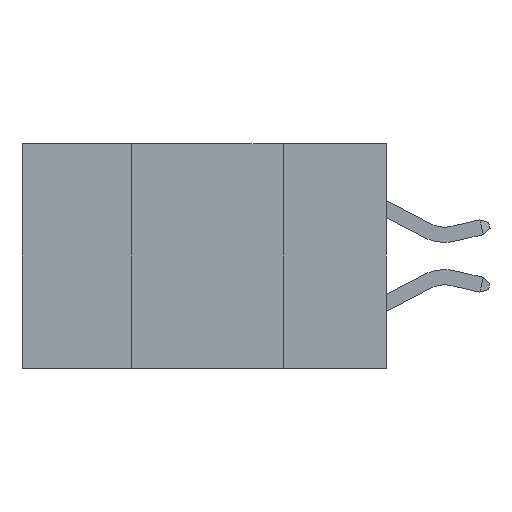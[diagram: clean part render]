
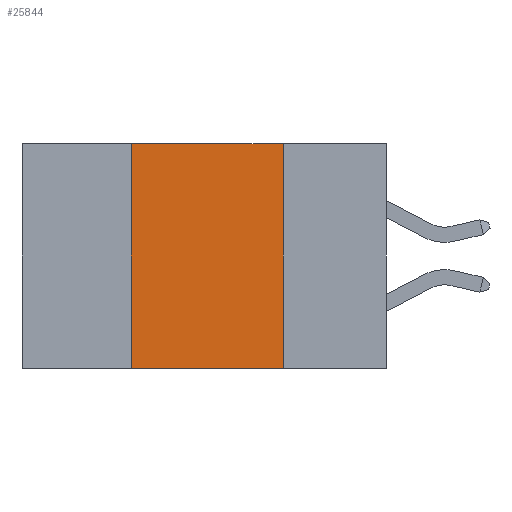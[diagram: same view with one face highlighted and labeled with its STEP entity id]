
A CAD part, left-side view. The second image highlights one B-rep face of the part: STEP entity #25844.
In plain terms, the highlighted planar face has unit normal (-1, 0, 0).
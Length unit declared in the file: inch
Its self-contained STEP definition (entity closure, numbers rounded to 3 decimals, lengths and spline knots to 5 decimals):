
#2453 = CARTESIAN_POINT ( 'NONE',  ( 0., 0.42, 0. ) ) ;
#2692 = VERTEX_POINT ( 'NONE', #3532 ) ;
#3270 = ORIENTED_EDGE ( 'NONE', *, *, #11109, .F. ) ;
#3532 = CARTESIAN_POINT ( 'NONE',  ( 0., 0.17, 0. ) ) ;
#4375 = ORIENTED_EDGE ( 'NONE', *, *, #20522, .F. ) ;
#4840 = DIRECTION ( 'NONE',  ( 0., 0., 1. ) ) ;
#5514 = LINE ( 'NONE', #24126, #29592 ) ;
#5540 = DIRECTION ( 'NONE',  ( 0., -1., 0. ) ) ;
#6798 = EDGE_CURVE ( 'NONE', #14443, #22079, #16952, .T. ) ;
#10240 = EDGE_LOOP ( 'NONE', ( #3270, #29569, #4375, #18853 ) ) ;
#10670 = CARTESIAN_POINT ( 'NONE',  ( 0., 0.17, 0. ) ) ;
#11109 = EDGE_CURVE ( 'NONE', #2692, #22079, #19258, .T. ) ;
#13027 = VECTOR ( 'NONE', #19995, 39.37008 ) ;
#13035 = DIRECTION ( 'NONE',  ( 0., 0., -1. ) ) ;
#13536 = EDGE_CURVE ( 'NONE', #14801, #2692, #5514, .T. ) ;
#14162 = FACE_OUTER_BOUND ( 'NONE', #10240, .T. ) ;
#14443 = VERTEX_POINT ( 'NONE', #21435 ) ;
#14801 = VERTEX_POINT ( 'NONE', #16130 ) ;
#15830 = LINE ( 'NONE', #2453, #27482 ) ;
#16130 = CARTESIAN_POINT ( 'NONE',  ( 0., 0.42, 0. ) ) ;
#16952 = LINE ( 'NONE', #24229, #21665 ) ;
#17229 = DIRECTION ( 'NONE',  ( 0., -1., 0. ) ) ;
#18853 = ORIENTED_EDGE ( 'NONE', *, *, #6798, .T. ) ;
#19258 = LINE ( 'NONE', #10670, #13027 ) ;
#19995 = DIRECTION ( 'NONE',  ( 0., 0., -1. ) ) ;
#20011 = CARTESIAN_POINT ( 'NONE',  ( 0., 0.6, 0. ) ) ;
#20522 = EDGE_CURVE ( 'NONE', #14443, #14801, #15830, .T. ) ;
#21435 = CARTESIAN_POINT ( 'NONE',  ( 0., 0.42, -0.37 ) ) ;
#21665 = VECTOR ( 'NONE', #5540, 39.37008 ) ;
#22079 = VERTEX_POINT ( 'NONE', #24486 ) ;
#24126 = CARTESIAN_POINT ( 'NONE',  ( 0., 0.6, 0. ) ) ;
#24229 = CARTESIAN_POINT ( 'NONE',  ( 0., 0.6, -0.37 ) ) ;
#24486 = CARTESIAN_POINT ( 'NONE',  ( 0., 0.17, -0.37 ) ) ;
#24752 = AXIS2_PLACEMENT_3D ( 'NONE', #20011, #26995, #13035 ) ;
#25844 = ADVANCED_FACE ( 'NONE', ( #14162 ), #29232, .F. ) ;
#26995 = DIRECTION ( 'NONE',  ( 1., 0., 0. ) ) ;
#27482 = VECTOR ( 'NONE', #4840, 39.37008 ) ;
#29232 = PLANE ( 'NONE',  #24752 ) ;
#29569 = ORIENTED_EDGE ( 'NONE', *, *, #13536, .F. ) ;
#29592 = VECTOR ( 'NONE', #17229, 39.37008 ) ;
